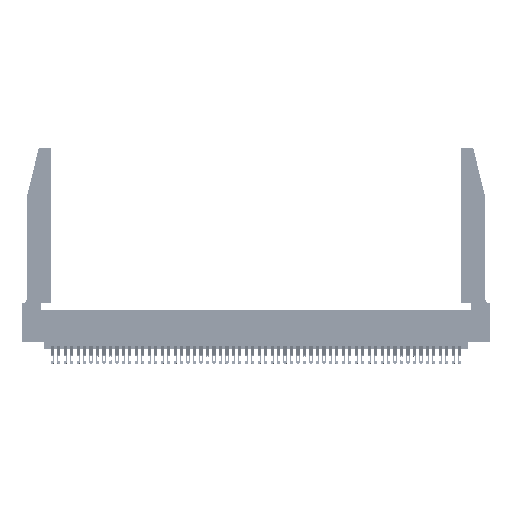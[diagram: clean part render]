
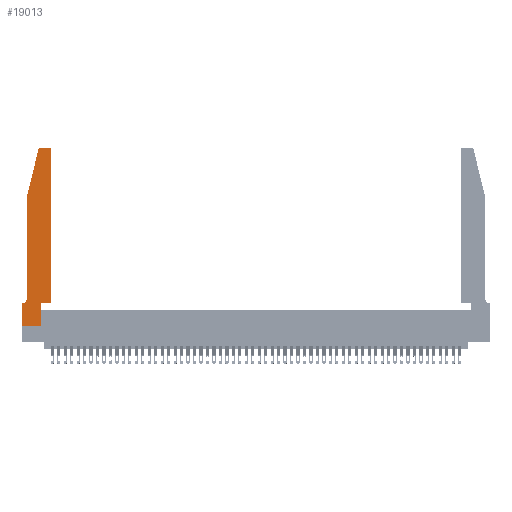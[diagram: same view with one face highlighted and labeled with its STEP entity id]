
A CAD part, top view. The second image highlights one B-rep face of the part: STEP entity #19013.
In plain terms, the highlighted planar face has unit normal (0, 0, 1).
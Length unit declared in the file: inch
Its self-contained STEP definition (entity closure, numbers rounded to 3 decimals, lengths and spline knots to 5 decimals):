
#386 = VERTEX_POINT ( 'NONE', #45042 ) ;
#405 = FACE_OUTER_BOUND ( 'NONE', #42641, .T. ) ;
#647 = CARTESIAN_POINT ( 'NONE',  ( 0.25487, 2.72718, 0.37 ) ) ;
#1037 = VERTEX_POINT ( 'NONE', #49751 ) ;
#1119 = CARTESIAN_POINT ( 'NONE',  ( 0.2865, 0.35, 0.37 ) ) ;
#1335 = LINE ( 'NONE', #16464, #26007 ) ;
#1746 = VERTEX_POINT ( 'NONE', #647 ) ;
#1959 = CARTESIAN_POINT ( 'NONE',  ( 0., 0.35, 0.37 ) ) ;
#2358 = VECTOR ( 'NONE', #25160, 39.37008 ) ;
#2770 = ORIENTED_EDGE ( 'NONE', *, *, #31459, .T. ) ;
#3434 = DIRECTION ( 'NONE',  ( -1., 0., 0. ) ) ;
#3502 = LINE ( 'NONE', #27277, #14867 ) ;
#3706 = CARTESIAN_POINT ( 'NONE',  ( 0.4505, 0.35, 0.37 ) ) ;
#4098 = DIRECTION ( 'NONE',  ( 0., -1., 0. ) ) ;
#4981 = LINE ( 'NONE', #44157, #34633 ) ;
#5385 = EDGE_CURVE ( 'NONE', #50031, #51267, #41600, .T. ) ;
#6759 = ORIENTED_EDGE ( 'NONE', *, *, #16470, .T. ) ;
#7725 = DIRECTION ( 'NONE',  ( 1., 0., 0. ) ) ;
#7977 = ORIENTED_EDGE ( 'NONE', *, *, #50707, .T. ) ;
#8070 = VERTEX_POINT ( 'NONE', #1959 ) ;
#9519 = VECTOR ( 'NONE', #48951, 39.37008 ) ;
#10504 = VERTEX_POINT ( 'NONE', #18481 ) ;
#10505 = AXIS2_PLACEMENT_3D ( 'NONE', #18776, #47123, #39296 ) ;
#10939 = CARTESIAN_POINT ( 'NONE',  ( 0.4505, 2.72, 0.37 ) ) ;
#12420 = EDGE_CURVE ( 'NONE', #10504, #8070, #51437, .T. ) ;
#13007 = VECTOR ( 'NONE', #16739, 39.37008 ) ;
#13356 = LINE ( 'NONE', #3706, #33557 ) ;
#14731 = ORIENTED_EDGE ( 'NONE', *, *, #12420, .T. ) ;
#14856 = CIRCLE ( 'NONE', #18882, 0.07 ) ;
#14867 = VECTOR ( 'NONE', #35729, 39.37008 ) ;
#14917 = CARTESIAN_POINT ( 'NONE',  ( 0.2605, 2.75, 0.37 ) ) ;
#15267 = DIRECTION ( 'NONE',  ( -1., 0., 0. ) ) ;
#15859 = CARTESIAN_POINT ( 'NONE',  ( 0.2865, 0.35, 0.37 ) ) ;
#16464 = CARTESIAN_POINT ( 'NONE',  ( 0., 0., 0.37 ) ) ;
#16470 = EDGE_CURVE ( 'NONE', #1037, #50031, #3502, .T. ) ;
#16659 = ORIENTED_EDGE ( 'NONE', *, *, #21825, .T. ) ;
#16739 = DIRECTION ( 'NONE',  ( 0., -1., 0. ) ) ;
#17150 = VECTOR ( 'NONE', #15267, 39.37008 ) ;
#17762 = VERTEX_POINT ( 'NONE', #36620 ) ;
#17875 = CARTESIAN_POINT ( 'NONE',  ( 0.0755, 2., 0.37 ) ) ;
#18481 = CARTESIAN_POINT ( 'NONE',  ( 0.0055, 0.35, 0.37 ) ) ;
#18776 = CARTESIAN_POINT ( 'NONE',  ( 0.284, 2.72, 0.37 ) ) ;
#18882 = AXIS2_PLACEMENT_3D ( 'NONE', #35237, #43064, #3434 ) ;
#19013 = ADVANCED_FACE ( 'NONE', ( #405 ), #36013, .T. ) ;
#19777 = DIRECTION ( 'NONE',  ( 1., 0., 0. ) ) ;
#20159 = CARTESIAN_POINT ( 'NONE',  ( 0.284, 2.75, 0.37 ) ) ;
#20689 = ORIENTED_EDGE ( 'NONE', *, *, #44310, .T. ) ;
#21484 = CARTESIAN_POINT ( 'NONE',  ( 0.2865, 0., 0.37 ) ) ;
#21825 = EDGE_CURVE ( 'NONE', #8070, #386, #1335, .T. ) ;
#22947 = ORIENTED_EDGE ( 'NONE', *, *, #5385, .T. ) ;
#24028 = DIRECTION ( 'NONE',  ( 0., 0., 1. ) ) ;
#24735 = LINE ( 'NONE', #1119, #9519 ) ;
#25160 = DIRECTION ( 'NONE',  ( -0.239, -0.971, 0. ) ) ;
#25866 = VERTEX_POINT ( 'NONE', #15859 ) ;
#26007 = VECTOR ( 'NONE', #4098, 39.37008 ) ;
#27277 = CARTESIAN_POINT ( 'NONE',  ( 0.4505, 0.35, 0.37 ) ) ;
#28769 = CARTESIAN_POINT ( 'NONE',  ( 0.0755, 0.35, 0.37 ) ) ;
#29004 = AXIS2_PLACEMENT_3D ( 'NONE', #52389, #48297, #32294 ) ;
#29540 = ORIENTED_EDGE ( 'NONE', *, *, #42198, .T. ) ;
#30425 = LINE ( 'NONE', #14917, #17150 ) ;
#31459 = EDGE_CURVE ( 'NONE', #35061, #25866, #24735, .T. ) ;
#32294 = DIRECTION ( 'NONE',  ( 1., 0., 0. ) ) ;
#32315 = AXIS2_PLACEMENT_3D ( 'NONE', #47770, #24028, #19777 ) ;
#32547 = VERTEX_POINT ( 'NONE', #20159 ) ;
#33096 = EDGE_CURVE ( 'NONE', #386, #35061, #4981, .T. ) ;
#33557 = VECTOR ( 'NONE', #7725, 39.37008 ) ;
#34633 = VECTOR ( 'NONE', #52008, 39.37008 ) ;
#35061 = VERTEX_POINT ( 'NONE', #21484 ) ;
#35237 = CARTESIAN_POINT ( 'NONE',  ( 0.0055, 0.42, 0.37 ) ) ;
#35729 = DIRECTION ( 'NONE',  ( 0., 1., 0. ) ) ;
#36013 = PLANE ( 'NONE',  #29004 ) ;
#36620 = CARTESIAN_POINT ( 'NONE',  ( 0.0755, 0.42, 0.37 ) ) ;
#37266 = EDGE_CURVE ( 'NONE', #51267, #32547, #30425, .T. ) ;
#39296 = DIRECTION ( 'NONE',  ( 1., 0., 0. ) ) ;
#39470 = EDGE_CURVE ( 'NONE', #1746, #51040, #46703, .T. ) ;
#41212 = CARTESIAN_POINT ( 'NONE',  ( 0.0755, 2., 0.37 ) ) ;
#41600 = CIRCLE ( 'NONE', #32315, 0.03 ) ;
#42198 = EDGE_CURVE ( 'NONE', #32547, #1746, #50807, .T. ) ;
#42641 = EDGE_LOOP ( 'NONE', ( #43258, #29540, #43296, #44348, #7977, #14731, #16659, #51497, #2770, #20689, #6759, #22947 ) ) ;
#43064 = DIRECTION ( 'NONE',  ( 0., 0., -1. ) ) ;
#43258 = ORIENTED_EDGE ( 'NONE', *, *, #37266, .T. ) ;
#43296 = ORIENTED_EDGE ( 'NONE', *, *, #39470, .T. ) ;
#44157 = CARTESIAN_POINT ( 'NONE',  ( 0., 0., 0.37 ) ) ;
#44189 = DIRECTION ( 'NONE',  ( -1., 0., 0. ) ) ;
#44310 = EDGE_CURVE ( 'NONE', #25866, #1037, #13356, .T. ) ;
#44348 = ORIENTED_EDGE ( 'NONE', *, *, #50333, .T. ) ;
#45042 = CARTESIAN_POINT ( 'NONE',  ( 0., 0., 0.37 ) ) ;
#45300 = LINE ( 'NONE', #48625, #13007 ) ;
#45709 = VECTOR ( 'NONE', #44189, 39.37008 ) ;
#46703 = LINE ( 'NONE', #41212, #2358 ) ;
#46750 = CARTESIAN_POINT ( 'NONE',  ( 0.4205, 2.75, 0.37 ) ) ;
#47123 = DIRECTION ( 'NONE',  ( 0., 0., 1. ) ) ;
#47770 = CARTESIAN_POINT ( 'NONE',  ( 0.4205, 2.72, 0.37 ) ) ;
#48297 = DIRECTION ( 'NONE',  ( 0., 0., 1. ) ) ;
#48625 = CARTESIAN_POINT ( 'NONE',  ( 0.0755, 2., 0.37 ) ) ;
#48951 = DIRECTION ( 'NONE',  ( 0., 1., 0. ) ) ;
#49751 = CARTESIAN_POINT ( 'NONE',  ( 0.4505, 0.35, 0.37 ) ) ;
#50031 = VERTEX_POINT ( 'NONE', #10939 ) ;
#50333 = EDGE_CURVE ( 'NONE', #51040, #17762, #45300, .T. ) ;
#50707 = EDGE_CURVE ( 'NONE', #17762, #10504, #14856, .T. ) ;
#50807 = CIRCLE ( 'NONE', #10505, 0.03 ) ;
#51040 = VERTEX_POINT ( 'NONE', #17875 ) ;
#51267 = VERTEX_POINT ( 'NONE', #46750 ) ;
#51437 = LINE ( 'NONE', #28769, #45709 ) ;
#51497 = ORIENTED_EDGE ( 'NONE', *, *, #33096, .T. ) ;
#52008 = DIRECTION ( 'NONE',  ( 1., 0., 0. ) ) ;
#52389 = CARTESIAN_POINT ( 'NONE',  ( 0., 0.35, 0.37 ) ) ;
